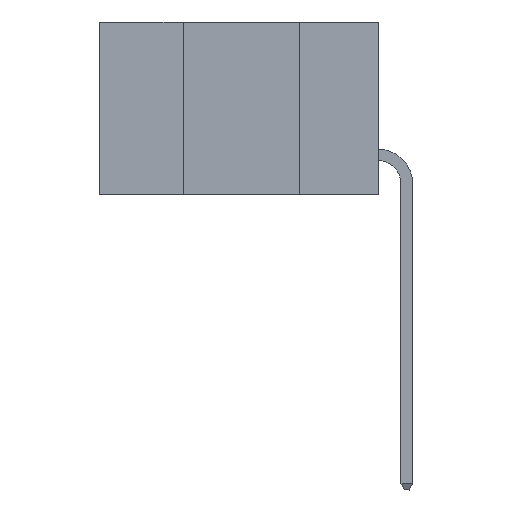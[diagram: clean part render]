
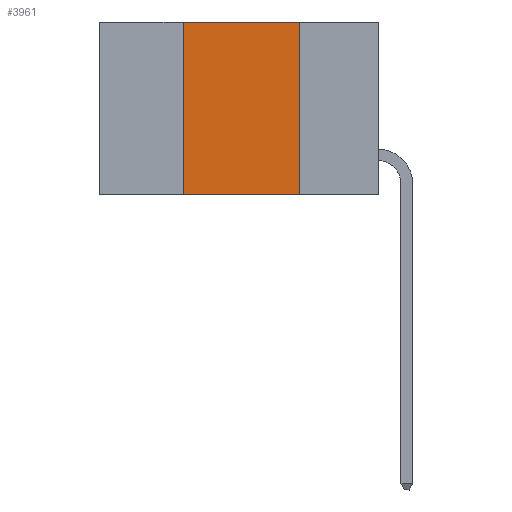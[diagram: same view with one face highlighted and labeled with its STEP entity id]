
A CAD part, left-side view. The second image highlights one B-rep face of the part: STEP entity #3961.
In plain terms, the highlighted planar face has unit normal (-1, 0, 0).
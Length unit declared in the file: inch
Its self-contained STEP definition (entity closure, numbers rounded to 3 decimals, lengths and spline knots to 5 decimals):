
#160 = DIRECTION ( 'NONE',  ( 0., -1., 0. ) ) ;
#258 = CARTESIAN_POINT ( 'NONE',  ( 0., 0.6, 0. ) ) ;
#480 = EDGE_CURVE ( 'NONE', #6280, #5195, #4355, .T. ) ;
#930 = DIRECTION ( 'NONE',  ( 0., 0., -1. ) ) ;
#1027 = LINE ( 'NONE', #258, #8257 ) ;
#1061 = EDGE_LOOP ( 'NONE', ( #1283, #8679, #8597, #8712 ) ) ;
#1283 = ORIENTED_EDGE ( 'NONE', *, *, #480, .F. ) ;
#1853 = CARTESIAN_POINT ( 'NONE',  ( 0., 0.42, -0.37 ) ) ;
#1904 = EDGE_CURVE ( 'NONE', #3934, #5195, #7436, .T. ) ;
#2401 = PLANE ( 'NONE',  #2690 ) ;
#2541 = CARTESIAN_POINT ( 'NONE',  ( 0., 0.6, 0. ) ) ;
#2690 = AXIS2_PLACEMENT_3D ( 'NONE', #2541, #8705, #8069 ) ;
#2835 = VECTOR ( 'NONE', #6060, 39.37008 ) ;
#2919 = VECTOR ( 'NONE', #930, 39.37008 ) ;
#3044 = CARTESIAN_POINT ( 'NONE',  ( 0., 0.42, 0. ) ) ;
#3308 = VECTOR ( 'NONE', #8916, 39.37008 ) ;
#3614 = LINE ( 'NONE', #7490, #3308 ) ;
#3934 = VERTEX_POINT ( 'NONE', #1853 ) ;
#3961 = ADVANCED_FACE ( 'NONE', ( #7466 ), #2401, .F. ) ;
#3997 = CARTESIAN_POINT ( 'NONE',  ( 0., 0.6, -0.37 ) ) ;
#4355 = LINE ( 'NONE', #4543, #2919 ) ;
#4497 = EDGE_CURVE ( 'NONE', #3934, #7732, #3614, .T. ) ;
#4543 = CARTESIAN_POINT ( 'NONE',  ( 0., 0.17, -0.37 ) ) ;
#4671 = EDGE_CURVE ( 'NONE', #7732, #6280, #1027, .T. ) ;
#5195 = VERTEX_POINT ( 'NONE', #7862 ) ;
#6060 = DIRECTION ( 'NONE',  ( 0., -1., 0. ) ) ;
#6140 = CARTESIAN_POINT ( 'NONE',  ( 0., 0.17, 0. ) ) ;
#6280 = VERTEX_POINT ( 'NONE', #6140 ) ;
#7436 = LINE ( 'NONE', #3997, #2835 ) ;
#7466 = FACE_OUTER_BOUND ( 'NONE', #1061, .T. ) ;
#7490 = CARTESIAN_POINT ( 'NONE',  ( 0., 0.42, -0.37 ) ) ;
#7732 = VERTEX_POINT ( 'NONE', #3044 ) ;
#7862 = CARTESIAN_POINT ( 'NONE',  ( 0., 0.17, -0.37 ) ) ;
#8069 = DIRECTION ( 'NONE',  ( 0., 0., -1. ) ) ;
#8257 = VECTOR ( 'NONE', #160, 39.37008 ) ;
#8597 = ORIENTED_EDGE ( 'NONE', *, *, #4497, .F. ) ;
#8679 = ORIENTED_EDGE ( 'NONE', *, *, #4671, .F. ) ;
#8705 = DIRECTION ( 'NONE',  ( 1., 0., 0. ) ) ;
#8712 = ORIENTED_EDGE ( 'NONE', *, *, #1904, .T. ) ;
#8916 = DIRECTION ( 'NONE',  ( 0., 0., 1. ) ) ;
